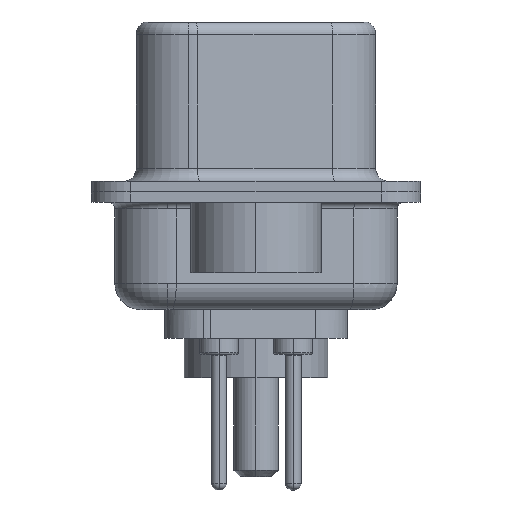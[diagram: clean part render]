
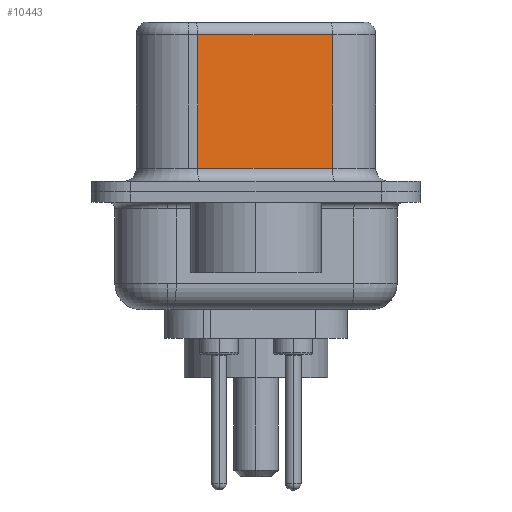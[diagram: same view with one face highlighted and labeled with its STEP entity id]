
A CAD part, left-side view. The second image highlights one B-rep face of the part: STEP entity #10443.
In plain terms, the highlighted planar face has unit normal (-0.985, -0.174, 0).
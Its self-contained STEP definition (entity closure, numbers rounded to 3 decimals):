
#1530 = DIRECTION ( 'NONE',  ( 0.174, -0.985, 0. ) ) ;
#1761 = VECTOR ( 'NONE', #13652, 1000. ) ;
#1888 = CARTESIAN_POINT ( 'NONE',  ( 4.565, -2.927, 0.9 ) ) ;
#2129 = DIRECTION ( 'NONE',  ( 0., 0., -1. ) ) ;
#2659 = EDGE_CURVE ( 'NONE', #12214, #10343, #15730, .T. ) ;
#3641 = DIRECTION ( 'NONE',  ( -0.174, 0.985, 0. ) ) ;
#4312 = CARTESIAN_POINT ( 'NONE',  ( 4.565, -2.927, 6.02 ) ) ;
#4476 = CARTESIAN_POINT ( 'NONE',  ( 3.655, 2.233, 6.52 ) ) ;
#4666 = FACE_OUTER_BOUND ( 'NONE', #8131, .T. ) ;
#6082 = DIRECTION ( 'NONE',  ( -0.174, 0.985, 0. ) ) ;
#6240 = ORIENTED_EDGE ( 'NONE', *, *, #7518, .T. ) ;
#7134 = AXIS2_PLACEMENT_3D ( 'NONE', #7338, #13886, #6082 ) ;
#7338 = CARTESIAN_POINT ( 'NONE',  ( 4.565, -2.927, 6.52 ) ) ;
#7518 = EDGE_CURVE ( 'NONE', #9104, #10773, #15776, .T. ) ;
#8131 = EDGE_LOOP ( 'NONE', ( #12380, #15862, #6240, #13580 ) ) ;
#8889 = EDGE_CURVE ( 'NONE', #12214, #9104, #9664, .T. ) ;
#9104 = VERTEX_POINT ( 'NONE', #15928 ) ;
#9496 = CARTESIAN_POINT ( 'NONE',  ( 4.565, -2.927, 0.9 ) ) ;
#9664 = LINE ( 'NONE', #15475, #16197 ) ;
#9766 = VECTOR ( 'NONE', #1530, 1000. ) ;
#10008 = PLANE ( 'NONE',  #7134 ) ;
#10343 = VERTEX_POINT ( 'NONE', #1888 ) ;
#10443 = ADVANCED_FACE ( 'NONE', ( #4666 ), #10008, .F. ) ;
#10773 = VERTEX_POINT ( 'NONE', #14405 ) ;
#12003 = CARTESIAN_POINT ( 'NONE',  ( 4.565, -2.927, 6.52 ) ) ;
#12214 = VERTEX_POINT ( 'NONE', #4312 ) ;
#12262 = VECTOR ( 'NONE', #2129, 1000. ) ;
#12380 = ORIENTED_EDGE ( 'NONE', *, *, #2659, .F. ) ;
#13190 = LINE ( 'NONE', #9496, #9766 ) ;
#13580 = ORIENTED_EDGE ( 'NONE', *, *, #15091, .T. ) ;
#13652 = DIRECTION ( 'NONE',  ( 0., 0., -1. ) ) ;
#13886 = DIRECTION ( 'NONE',  ( 0.985, 0.174, 0. ) ) ;
#14405 = CARTESIAN_POINT ( 'NONE',  ( 3.655, 2.233, 0.9 ) ) ;
#15091 = EDGE_CURVE ( 'NONE', #10773, #10343, #13190, .T. ) ;
#15475 = CARTESIAN_POINT ( 'NONE',  ( 4.565, -2.927, 6.02 ) ) ;
#15730 = LINE ( 'NONE', #12003, #12262 ) ;
#15776 = LINE ( 'NONE', #4476, #1761 ) ;
#15862 = ORIENTED_EDGE ( 'NONE', *, *, #8889, .T. ) ;
#15928 = CARTESIAN_POINT ( 'NONE',  ( 3.655, 2.233, 6.02 ) ) ;
#16197 = VECTOR ( 'NONE', #3641, 1000. ) ;
